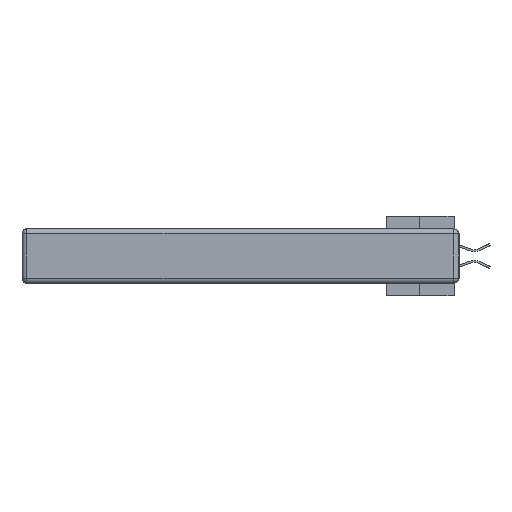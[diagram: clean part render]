
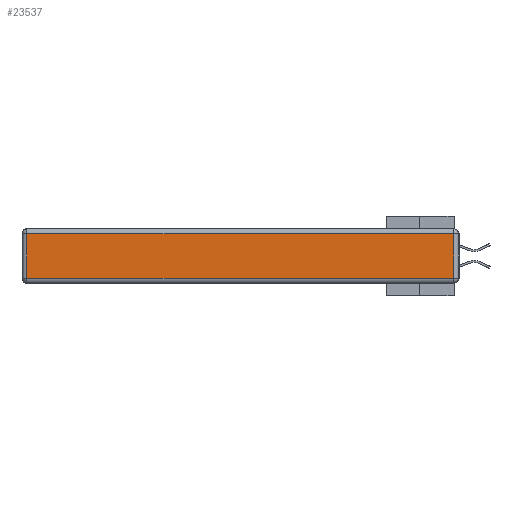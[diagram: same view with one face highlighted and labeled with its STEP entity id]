
A CAD part, left-side view. The second image highlights one B-rep face of the part: STEP entity #23537.
In plain terms, the highlighted planar face has unit normal (-1, 0, 0).
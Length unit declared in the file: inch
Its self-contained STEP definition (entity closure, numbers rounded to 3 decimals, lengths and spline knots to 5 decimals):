
#1465 = CARTESIAN_POINT ( 'NONE',  ( 0., 0.03, -0.313 ) ) ;
#2031 = CARTESIAN_POINT ( 'NONE',  ( 0., 0.03, -0.03 ) ) ;
#2827 = CARTESIAN_POINT ( 'NONE',  ( 0., 2.72, -0.343 ) ) ;
#4971 = VERTEX_POINT ( 'NONE', #5730 ) ;
#5730 = CARTESIAN_POINT ( 'NONE',  ( 0., 2.72, -0.313 ) ) ;
#5997 = VERTEX_POINT ( 'NONE', #2031 ) ;
#8044 = EDGE_CURVE ( 'NONE', #4971, #27504, #30315, .T. ) ;
#8081 = FACE_OUTER_BOUND ( 'NONE', #17307, .T. ) ;
#8525 = PLANE ( 'NONE',  #46347 ) ;
#8622 = EDGE_CURVE ( 'NONE', #26100, #4971, #13920, .T. ) ;
#8677 = VECTOR ( 'NONE', #31560, 39.37008 ) ;
#8692 = DIRECTION ( 'NONE',  ( -1., 0., 0. ) ) ;
#13920 = LINE ( 'NONE', #2827, #29689 ) ;
#15494 = DIRECTION ( 'NONE',  ( 0., 0., 1. ) ) ;
#17307 = EDGE_LOOP ( 'NONE', ( #39818, #41955, #42533, #36561 ) ) ;
#20776 = VECTOR ( 'NONE', #24488, 39.37008 ) ;
#22364 = CARTESIAN_POINT ( 'NONE',  ( 0., 2.72, -0.03 ) ) ;
#22885 = CARTESIAN_POINT ( 'NONE',  ( 0., 2.75, -0.03 ) ) ;
#23005 = EDGE_CURVE ( 'NONE', #27504, #5997, #24451, .T. ) ;
#23537 = ADVANCED_FACE ( 'NONE', ( #8081 ), #8525, .T. ) ;
#24451 = LINE ( 'NONE', #39054, #8677 ) ;
#24488 = DIRECTION ( 'NONE',  ( 0., -1., 0. ) ) ;
#26100 = VERTEX_POINT ( 'NONE', #22364 ) ;
#26716 = LINE ( 'NONE', #22885, #36783 ) ;
#27504 = VERTEX_POINT ( 'NONE', #1465 ) ;
#28306 = DIRECTION ( 'NONE',  ( 0., 0., -1. ) ) ;
#29689 = VECTOR ( 'NONE', #28306, 39.37008 ) ;
#30056 = DIRECTION ( 'NONE',  ( 0., 1., 0. ) ) ;
#30315 = LINE ( 'NONE', #39069, #20776 ) ;
#31560 = DIRECTION ( 'NONE',  ( 0., 0., 1. ) ) ;
#33473 = EDGE_CURVE ( 'NONE', #5997, #26100, #26716, .T. ) ;
#33852 = CARTESIAN_POINT ( 'NONE',  ( 0., 0., -0.343 ) ) ;
#36561 = ORIENTED_EDGE ( 'NONE', *, *, #8622, .T. ) ;
#36783 = VECTOR ( 'NONE', #30056, 39.37008 ) ;
#39054 = CARTESIAN_POINT ( 'NONE',  ( 0., 0.03, -0.343 ) ) ;
#39069 = CARTESIAN_POINT ( 'NONE',  ( 0., 0., -0.313 ) ) ;
#39818 = ORIENTED_EDGE ( 'NONE', *, *, #8044, .T. ) ;
#41955 = ORIENTED_EDGE ( 'NONE', *, *, #23005, .T. ) ;
#42533 = ORIENTED_EDGE ( 'NONE', *, *, #33473, .T. ) ;
#46347 = AXIS2_PLACEMENT_3D ( 'NONE', #33852, #8692, #15494 ) ;
